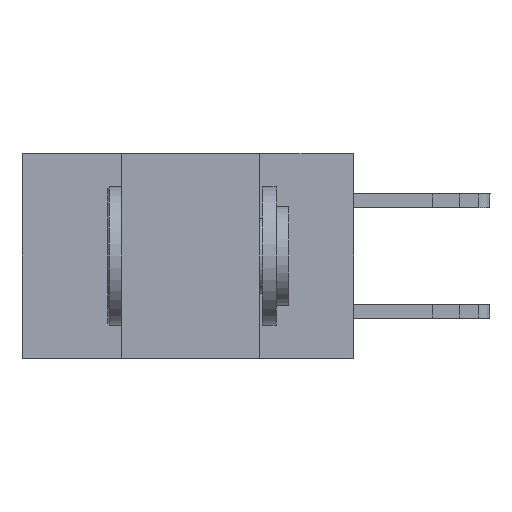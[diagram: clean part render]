
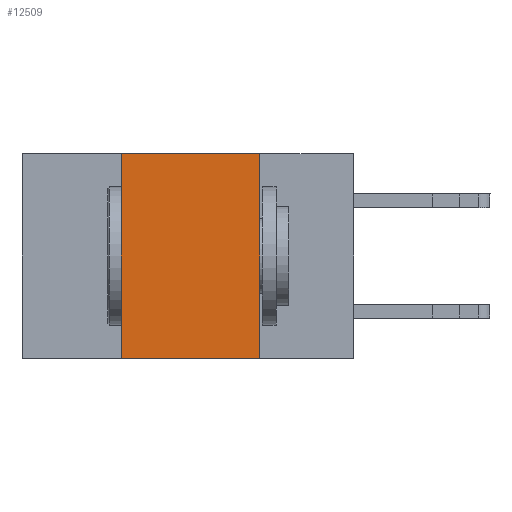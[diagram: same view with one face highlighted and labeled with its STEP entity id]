
A CAD part, left-side view. The second image highlights one B-rep face of the part: STEP entity #12509.
In plain terms, the highlighted planar face has unit normal (-1, 0, 0).
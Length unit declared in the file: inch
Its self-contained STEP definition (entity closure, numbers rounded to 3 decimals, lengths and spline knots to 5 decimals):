
#340 = DIRECTION ( 'NONE',  ( 0., -1., 0. ) ) ;
#1305 = VERTEX_POINT ( 'NONE', #15440 ) ;
#1743 = DIRECTION ( 'NONE',  ( 0., 0., -1. ) ) ;
#1970 = DIRECTION ( 'NONE',  ( 1., 0., 0. ) ) ;
#3258 = LINE ( 'NONE', #15469, #19989 ) ;
#4255 = AXIS2_PLACEMENT_3D ( 'NONE', #8646, #1970, #13624 ) ;
#5876 = DIRECTION ( 'NONE',  ( 0., -1., 0. ) ) ;
#6207 = DIRECTION ( 'NONE',  ( 0., 0., 1. ) ) ;
#8046 = CARTESIAN_POINT ( 'NONE',  ( 0., 0.42, 0. ) ) ;
#8214 = EDGE_CURVE ( 'NONE', #17431, #1305, #11809, .T. ) ;
#8238 = CARTESIAN_POINT ( 'NONE',  ( 0., 0.17, 0. ) ) ;
#8646 = CARTESIAN_POINT ( 'NONE',  ( 0., 0.6, 0. ) ) ;
#8703 = VECTOR ( 'NONE', #5876, 39.37008 ) ;
#9292 = EDGE_CURVE ( 'NONE', #12802, #15087, #18936, .T. ) ;
#9356 = CARTESIAN_POINT ( 'NONE',  ( 0., 0.17, 0. ) ) ;
#10024 = LINE ( 'NONE', #19351, #8703 ) ;
#11687 = EDGE_LOOP ( 'NONE', ( #14520, #19840, #17891, #20069 ) ) ;
#11809 = LINE ( 'NONE', #9356, #13140 ) ;
#12283 = VECTOR ( 'NONE', #6207, 39.37008 ) ;
#12509 = ADVANCED_FACE ( 'NONE', ( #20073 ), #17342, .F. ) ;
#12802 = VERTEX_POINT ( 'NONE', #15111 ) ;
#13140 = VECTOR ( 'NONE', #1743, 39.37008 ) ;
#13624 = DIRECTION ( 'NONE',  ( 0., 0., -1. ) ) ;
#14237 = CARTESIAN_POINT ( 'NONE',  ( 0., 0.42, 0. ) ) ;
#14520 = ORIENTED_EDGE ( 'NONE', *, *, #8214, .F. ) ;
#14659 = EDGE_CURVE ( 'NONE', #15087, #17431, #3258, .T. ) ;
#15087 = VERTEX_POINT ( 'NONE', #14237 ) ;
#15111 = CARTESIAN_POINT ( 'NONE',  ( 0., 0.42, -0.37 ) ) ;
#15440 = CARTESIAN_POINT ( 'NONE',  ( 0., 0.17, -0.37 ) ) ;
#15469 = CARTESIAN_POINT ( 'NONE',  ( 0., 0.6, 0. ) ) ;
#17342 = PLANE ( 'NONE',  #4255 ) ;
#17431 = VERTEX_POINT ( 'NONE', #8238 ) ;
#17891 = ORIENTED_EDGE ( 'NONE', *, *, #9292, .F. ) ;
#18295 = EDGE_CURVE ( 'NONE', #12802, #1305, #10024, .T. ) ;
#18936 = LINE ( 'NONE', #8046, #12283 ) ;
#19351 = CARTESIAN_POINT ( 'NONE',  ( 0., 0.6, -0.37 ) ) ;
#19840 = ORIENTED_EDGE ( 'NONE', *, *, #14659, .F. ) ;
#19989 = VECTOR ( 'NONE', #340, 39.37008 ) ;
#20069 = ORIENTED_EDGE ( 'NONE', *, *, #18295, .T. ) ;
#20073 = FACE_OUTER_BOUND ( 'NONE', #11687, .T. ) ;
